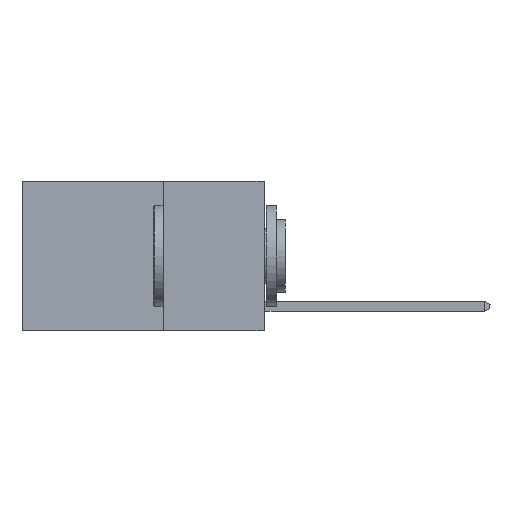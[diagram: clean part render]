
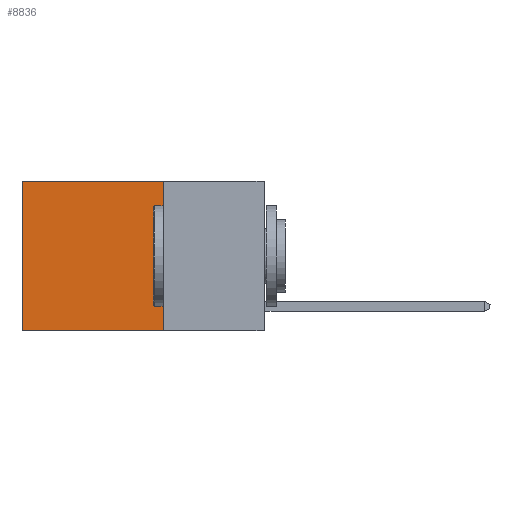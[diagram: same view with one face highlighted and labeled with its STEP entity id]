
A CAD part, left-side view. The second image highlights one B-rep face of the part: STEP entity #8836.
In plain terms, the highlighted planar face has unit normal (-1, 0, 0).
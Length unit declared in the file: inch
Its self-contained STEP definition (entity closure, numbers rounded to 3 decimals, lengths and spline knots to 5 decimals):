
#573 = VERTEX_POINT ( 'NONE', #13330 ) ;
#1653 = ORIENTED_EDGE ( 'NONE', *, *, #13312, .F. ) ;
#2457 = DIRECTION ( 'NONE',  ( 0., 1., 0. ) ) ;
#3055 = VECTOR ( 'NONE', #7666, 39.37008 ) ;
#3269 = DIRECTION ( 'NONE',  ( 0., 0., -1. ) ) ;
#3934 = ORIENTED_EDGE ( 'NONE', *, *, #15389, .T. ) ;
#3936 = LINE ( 'NONE', #17478, #6858 ) ;
#4811 = DIRECTION ( 'NONE',  ( 0., 0., -1. ) ) ;
#6108 = CARTESIAN_POINT ( 'NONE',  ( 0.2625, 0.25, 0. ) ) ;
#6192 = FACE_OUTER_BOUND ( 'NONE', #12054, .T. ) ;
#6506 = VERTEX_POINT ( 'NONE', #18868 ) ;
#6858 = VECTOR ( 'NONE', #2457, 39.37008 ) ;
#7376 = EDGE_CURVE ( 'NONE', #9760, #573, #3936, .T. ) ;
#7666 = DIRECTION ( 'NONE',  ( 0., 0., -1. ) ) ;
#7794 = CARTESIAN_POINT ( 'NONE',  ( 0.2625, 0.25, 0. ) ) ;
#8046 = LINE ( 'NONE', #18163, #3055 ) ;
#8836 = ADVANCED_FACE ( 'NONE', ( #6192 ), #10309, .F. ) ;
#8849 = LINE ( 'NONE', #6108, #18663 ) ;
#9343 = ORIENTED_EDGE ( 'NONE', *, *, #7376, .F. ) ;
#9760 = VERTEX_POINT ( 'NONE', #12212 ) ;
#10309 = PLANE ( 'NONE',  #17379 ) ;
#10985 = DIRECTION ( 'NONE',  ( 1., 0., 0. ) ) ;
#12054 = EDGE_LOOP ( 'NONE', ( #3934, #9343, #1653, #14913 ) ) ;
#12212 = CARTESIAN_POINT ( 'NONE',  ( 0.2625, 0.25, -0.37 ) ) ;
#12305 = EDGE_CURVE ( 'NONE', #17400, #6506, #8849, .T. ) ;
#12495 = LINE ( 'NONE', #7794, #17428 ) ;
#13312 = EDGE_CURVE ( 'NONE', #17400, #9760, #12495, .T. ) ;
#13330 = CARTESIAN_POINT ( 'NONE',  ( 0.2625, 0.6, -0.37 ) ) ;
#13590 = CARTESIAN_POINT ( 'NONE',  ( 0.2625, 0.25, 0. ) ) ;
#14913 = ORIENTED_EDGE ( 'NONE', *, *, #12305, .T. ) ;
#15389 = EDGE_CURVE ( 'NONE', #6506, #573, #8046, .T. ) ;
#17379 = AXIS2_PLACEMENT_3D ( 'NONE', #18153, #10985, #4811 ) ;
#17400 = VERTEX_POINT ( 'NONE', #13590 ) ;
#17428 = VECTOR ( 'NONE', #3269, 39.37008 ) ;
#17478 = CARTESIAN_POINT ( 'NONE',  ( 0.2625, 0.25, -0.37 ) ) ;
#18153 = CARTESIAN_POINT ( 'NONE',  ( 0.2625, 0.25, 0. ) ) ;
#18163 = CARTESIAN_POINT ( 'NONE',  ( 0.2625, 0.6, 0. ) ) ;
#18663 = VECTOR ( 'NONE', #19256, 39.37008 ) ;
#18868 = CARTESIAN_POINT ( 'NONE',  ( 0.2625, 0.6, 0. ) ) ;
#19256 = DIRECTION ( 'NONE',  ( 0., 1., 0. ) ) ;
